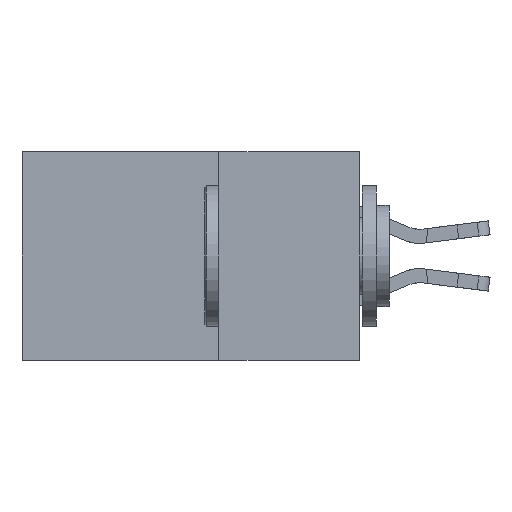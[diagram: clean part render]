
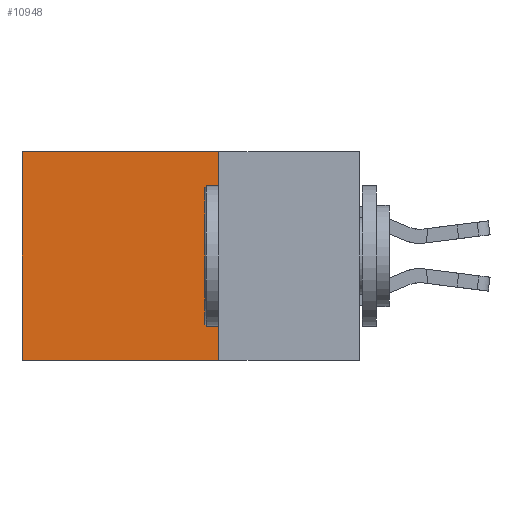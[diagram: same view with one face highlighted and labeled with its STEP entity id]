
A CAD part, left-side view. The second image highlights one B-rep face of the part: STEP entity #10948.
In plain terms, the highlighted planar face has unit normal (-1, 0, 0).
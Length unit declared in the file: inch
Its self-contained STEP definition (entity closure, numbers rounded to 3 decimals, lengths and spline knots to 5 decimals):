
#86 = VECTOR ( 'NONE', #23191, 39.37008 ) ;
#329 = ORIENTED_EDGE ( 'NONE', *, *, #6749, .F. ) ;
#1240 = LINE ( 'NONE', #10268, #86 ) ;
#2548 = EDGE_CURVE ( 'NONE', #7772, #5525, #11353, .T. ) ;
#3238 = FACE_OUTER_BOUND ( 'NONE', #21648, .T. ) ;
#3360 = CARTESIAN_POINT ( 'NONE',  ( 0.2875, 0.25, 0. ) ) ;
#3475 = CARTESIAN_POINT ( 'NONE',  ( 0.2875, 0.25, -0.37 ) ) ;
#4998 = ORIENTED_EDGE ( 'NONE', *, *, #19333, .T. ) ;
#5525 = VERTEX_POINT ( 'NONE', #21071 ) ;
#6362 = ORIENTED_EDGE ( 'NONE', *, *, #7146, .T. ) ;
#6509 = CARTESIAN_POINT ( 'NONE',  ( 0.2875, 0.25, -0.37 ) ) ;
#6747 = DIRECTION ( 'NONE',  ( 0., 1., 0. ) ) ;
#6749 = EDGE_CURVE ( 'NONE', #16979, #7772, #19932, .T. ) ;
#7076 = DIRECTION ( 'NONE',  ( 0., 0., -1. ) ) ;
#7146 = EDGE_CURVE ( 'NONE', #22382, #5525, #11957, .T. ) ;
#7772 = VERTEX_POINT ( 'NONE', #3475 ) ;
#8556 = VECTOR ( 'NONE', #10218, 39.37008 ) ;
#10218 = DIRECTION ( 'NONE',  ( 0., 0., -1. ) ) ;
#10268 = CARTESIAN_POINT ( 'NONE',  ( 0.2875, 0.25, 0. ) ) ;
#10566 = VECTOR ( 'NONE', #7076, 39.37008 ) ;
#10948 = ADVANCED_FACE ( 'NONE', ( #3238 ), #16478, .F. ) ;
#11177 = CARTESIAN_POINT ( 'NONE',  ( 0.2875, 0.25, 0. ) ) ;
#11261 = DIRECTION ( 'NONE',  ( 1., 0., 0. ) ) ;
#11353 = LINE ( 'NONE', #6509, #12761 ) ;
#11957 = LINE ( 'NONE', #14089, #8556 ) ;
#12761 = VECTOR ( 'NONE', #6747, 39.37008 ) ;
#14089 = CARTESIAN_POINT ( 'NONE',  ( 0.2875, 0.6, 0. ) ) ;
#15872 = CARTESIAN_POINT ( 'NONE',  ( 0.2875, 0.25, 0. ) ) ;
#16478 = PLANE ( 'NONE',  #20115 ) ;
#16979 = VERTEX_POINT ( 'NONE', #15872 ) ;
#18214 = DIRECTION ( 'NONE',  ( 0., 0., -1. ) ) ;
#18599 = CARTESIAN_POINT ( 'NONE',  ( 0.2875, 0.6, 0. ) ) ;
#19333 = EDGE_CURVE ( 'NONE', #16979, #22382, #1240, .T. ) ;
#19709 = ORIENTED_EDGE ( 'NONE', *, *, #2548, .F. ) ;
#19932 = LINE ( 'NONE', #3360, #10566 ) ;
#20115 = AXIS2_PLACEMENT_3D ( 'NONE', #11177, #11261, #18214 ) ;
#21071 = CARTESIAN_POINT ( 'NONE',  ( 0.2875, 0.6, -0.37 ) ) ;
#21648 = EDGE_LOOP ( 'NONE', ( #6362, #19709, #329, #4998 ) ) ;
#22382 = VERTEX_POINT ( 'NONE', #18599 ) ;
#23191 = DIRECTION ( 'NONE',  ( 0., 1., 0. ) ) ;
